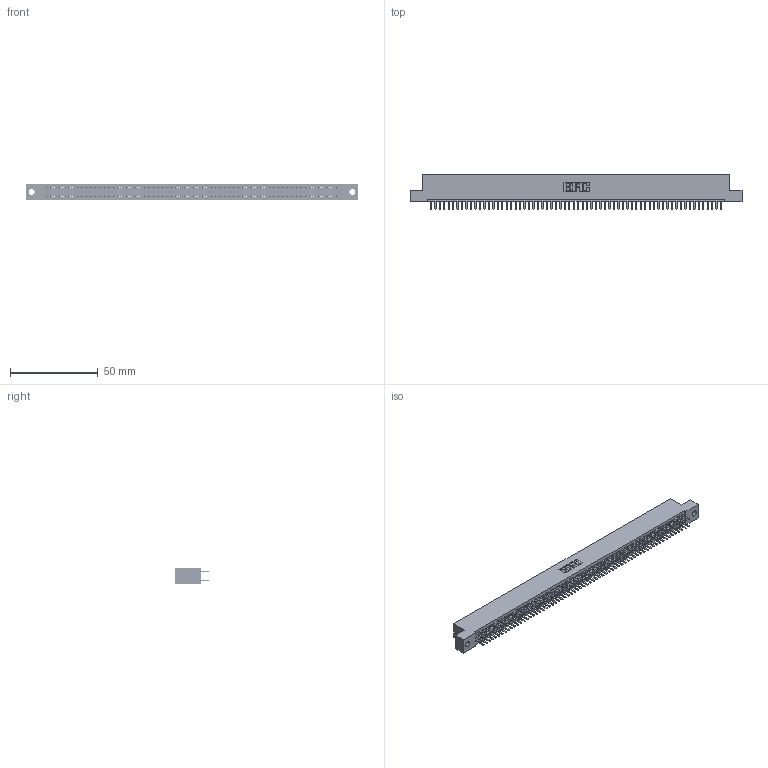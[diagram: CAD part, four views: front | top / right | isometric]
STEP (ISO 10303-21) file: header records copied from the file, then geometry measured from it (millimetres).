
FILE_DESCRIPTION (( 'STEP AP203' ), '1' );
FILE_NAME ('345-132-520-202.STEP', '2019-11-07T18:23:13', ( '' ), ( '' ), 'SwSTEP 2.0', 'SolidWorks 2016', '' );
FILE_SCHEMA (( 'CONFIG_CONTROL_DESIGN' ));
Length unit declared in the file: inch
Products named in the file (3): 345-132-520-202; 345-292-001_345-293-120; 345 Part_Flush Mounting Lugs - 0.128 Dia
Assembly tree (133 placements, depth 2):
  345-132-520-202
    345 Part_Flush Mounting Lugs - 0.128 Dia
    345-292-001_345-293-120  x132
Bounding box: 188.85 x 19.68 x 9.4 mm (x, y, z)
Volume: 18473 mm3; surface area: 27375 mm2
Topology: 133 solids, 133 shells, 7254 faces, 21065 edges, 13690 vertices
Faces by surface type: plane 4700, cylinder 2554
Entity records: 48671 total; most frequent: CARTESIAN_POINT 8148, ORIENTED_EDGE 8070, DIRECTION 7143, EDGE_CURVE 4035, VECTOR 3635, LINE 3635, VERTEX_POINT 2686, AXIS2_PLACEMENT_3D 1754
